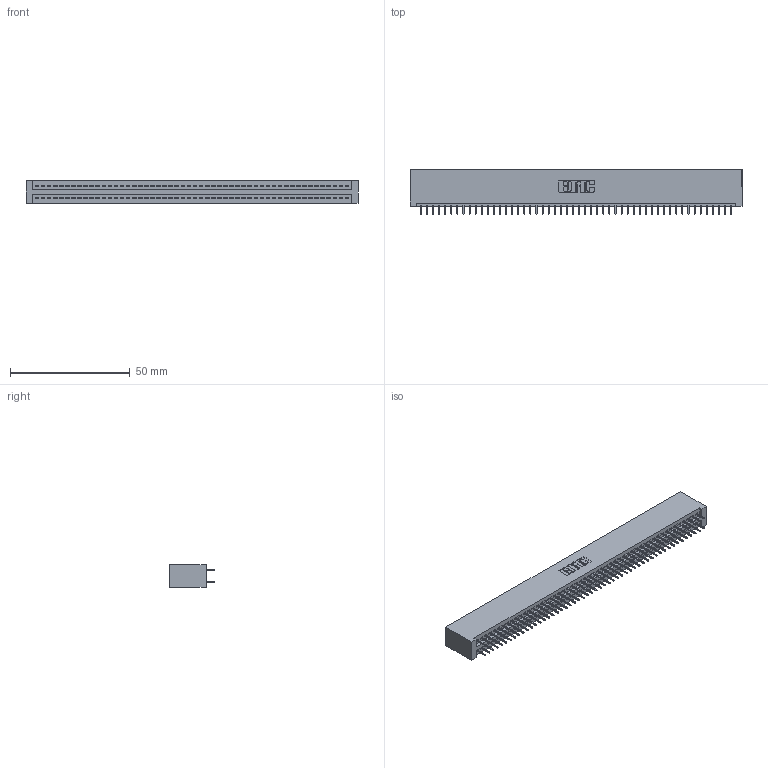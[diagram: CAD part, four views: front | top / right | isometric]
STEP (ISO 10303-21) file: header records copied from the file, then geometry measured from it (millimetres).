
FILE_DESCRIPTION (( 'STEP AP203' ), '1' );
FILE_NAME ('345-104-525-201.STEP', '2020-09-21T19:06:05', ( '' ), ( '' ), 'SwSTEP 2.0', 'SolidWorks 2020', '' );
FILE_SCHEMA (( 'CONFIG_CONTROL_DESIGN' ));
Length unit declared in the file: inch
Products named in the file (3): 345-292-001_345-293-125; 345-104-525-201; 345 Part_No Mounting Lugs
Assembly tree (105 placements, depth 2):
  345-104-525-201
    345 Part_No Mounting Lugs
    345-292-001_345-293-125  x104
Bounding box: 138.68 x 18.72 x 9.4 mm (x, y, z)
Volume: 14009.4 mm3; surface area: 20689.4 mm2
Topology: 105 solids, 105 shells, 5734 faces, 16229 edges, 10402 vertices
Faces by surface type: plane 4132, cylinder 1602
Entity records: 39251 total; most frequent: CARTESIAN_POINT 6568, ORIENTED_EDGE 6502, DIRECTION 5775, EDGE_CURVE 3251, VECTOR 2923, LINE 2923, VERTEX_POINT 2162, AXIS2_PLACEMENT_3D 1426
